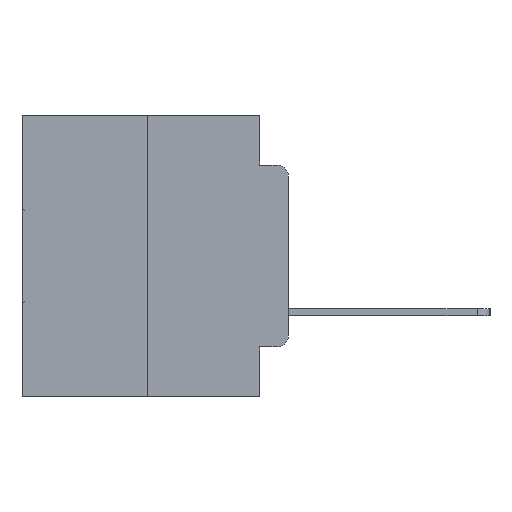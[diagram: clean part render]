
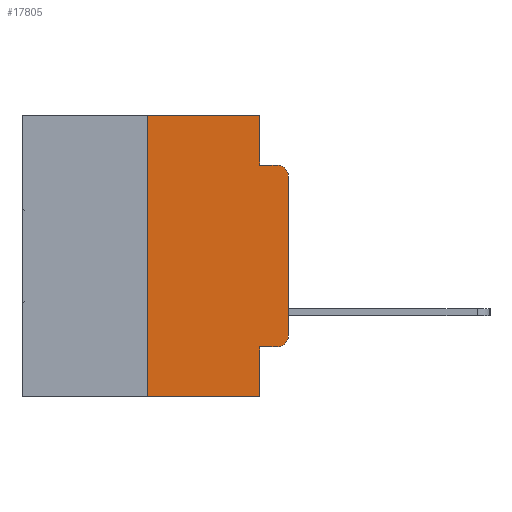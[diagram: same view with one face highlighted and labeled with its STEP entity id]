
A CAD part, left-side view. The second image highlights one B-rep face of the part: STEP entity #17805.
In plain terms, the highlighted planar face has unit normal (-1, 0, 0).
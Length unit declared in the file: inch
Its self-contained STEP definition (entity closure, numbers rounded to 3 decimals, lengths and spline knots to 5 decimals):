
#22 = DIRECTION ( 'NONE',  ( 0., -1., 0. ) ) ;
#305 = EDGE_CURVE ( 'NONE', #5735, #584, #22031, .T. ) ;
#584 = VERTEX_POINT ( 'NONE', #6001 ) ;
#732 = CARTESIAN_POINT ( 'NONE',  ( 0., 0., 0. ) ) ;
#795 = DIRECTION ( 'NONE',  ( 0., 0., -1. ) ) ;
#1579 = LINE ( 'NONE', #11698, #13246 ) ;
#1868 = DIRECTION ( 'NONE',  ( 0., 0., -1. ) ) ;
#2192 = CARTESIAN_POINT ( 'NONE',  ( 0., 0.051, -0.4115 ) ) ;
#2317 = EDGE_CURVE ( 'NONE', #20866, #5735, #18173, .T. ) ;
#2968 = VERTEX_POINT ( 'NONE', #26319 ) ;
#3524 = DIRECTION ( 'NONE',  ( 0., -1., 0. ) ) ;
#3721 = VECTOR ( 'NONE', #23520, 39.37008 ) ;
#3777 = AXIS2_PLACEMENT_3D ( 'NONE', #26623, #26662, #23555 ) ;
#3872 = EDGE_CURVE ( 'NONE', #2968, #20866, #18492, .T. ) ;
#4192 = CARTESIAN_POINT ( 'NONE',  ( 0., 0.051, 0. ) ) ;
#4450 = VERTEX_POINT ( 'NONE', #26108 ) ;
#4861 = DIRECTION ( 'NONE',  ( 0., 0., -1. ) ) ;
#5100 = LINE ( 'NONE', #16419, #10590 ) ;
#5735 = VERTEX_POINT ( 'NONE', #8322 ) ;
#6001 = CARTESIAN_POINT ( 'NONE',  ( 0., 0., -0.1085 ) ) ;
#6423 = AXIS2_PLACEMENT_3D ( 'NONE', #16955, #14727, #795 ) ;
#6938 = CARTESIAN_POINT ( 'NONE',  ( 0., 0.051, -0.5 ) ) ;
#7175 = EDGE_LOOP ( 'NONE', ( #10568, #18130, #8003, #26688, #22268, #17783, #13132, #14548, #16024, #17432 ) ) ;
#7553 = EDGE_CURVE ( 'NONE', #26560, #16601, #14676, .T. ) ;
#7652 = CARTESIAN_POINT ( 'NONE',  ( 0., 0.473, 0. ) ) ;
#7906 = AXIS2_PLACEMENT_3D ( 'NONE', #28959, #15793, #1868 ) ;
#8003 = ORIENTED_EDGE ( 'NONE', *, *, #7553, .F. ) ;
#8322 = CARTESIAN_POINT ( 'NONE',  ( 0., 0., -0.3915 ) ) ;
#9717 = CARTESIAN_POINT ( 'NONE',  ( 0., 0.25, 0. ) ) ;
#9956 = VECTOR ( 'NONE', #24204, 39.37008 ) ;
#10568 = ORIENTED_EDGE ( 'NONE', *, *, #305, .T. ) ;
#10590 = VECTOR ( 'NONE', #4861, 39.37008 ) ;
#11087 = CARTESIAN_POINT ( 'NONE',  ( 0., 0.25, 0. ) ) ;
#11698 = CARTESIAN_POINT ( 'NONE',  ( 0., 0.473, -0.5 ) ) ;
#11951 = VECTOR ( 'NONE', #22477, 39.37008 ) ;
#12445 = PLANE ( 'NONE',  #6423 ) ;
#13132 = ORIENTED_EDGE ( 'NONE', *, *, #25888, .T. ) ;
#13246 = VECTOR ( 'NONE', #22, 39.37008 ) ;
#13635 = VECTOR ( 'NONE', #26700, 39.37008 ) ;
#14115 = LINE ( 'NONE', #4192, #11951 ) ;
#14208 = VERTEX_POINT ( 'NONE', #6938 ) ;
#14324 = LINE ( 'NONE', #11087, #13635 ) ;
#14464 = FACE_OUTER_BOUND ( 'NONE', #7175, .T. ) ;
#14548 = ORIENTED_EDGE ( 'NONE', *, *, #18091, .F. ) ;
#14676 = LINE ( 'NONE', #20909, #20699 ) ;
#14727 = DIRECTION ( 'NONE',  ( 1., 0., 0. ) ) ;
#15328 = EDGE_CURVE ( 'NONE', #584, #16601, #27439, .T. ) ;
#15566 = EDGE_CURVE ( 'NONE', #28859, #19175, #21282, .T. ) ;
#15595 = CARTESIAN_POINT ( 'NONE',  ( 0., 0.02, -0.4115 ) ) ;
#15793 = DIRECTION ( 'NONE',  ( -1., 0., 0. ) ) ;
#16024 = ORIENTED_EDGE ( 'NONE', *, *, #3872, .T. ) ;
#16362 = CARTESIAN_POINT ( 'NONE',  ( 0., 0.051, -0.0885 ) ) ;
#16419 = CARTESIAN_POINT ( 'NONE',  ( 0., 0.051, 0. ) ) ;
#16601 = VERTEX_POINT ( 'NONE', #27849 ) ;
#16955 = CARTESIAN_POINT ( 'NONE',  ( 0., 0.473, 0. ) ) ;
#17432 = ORIENTED_EDGE ( 'NONE', *, *, #2317, .T. ) ;
#17783 = ORIENTED_EDGE ( 'NONE', *, *, #25730, .F. ) ;
#17792 = VECTOR ( 'NONE', #3524, 39.37008 ) ;
#17805 = ADVANCED_FACE ( 'NONE', ( #14464 ), #12445, .F. ) ;
#18091 = EDGE_CURVE ( 'NONE', #2968, #14208, #14115, .T. ) ;
#18130 = ORIENTED_EDGE ( 'NONE', *, *, #15328, .T. ) ;
#18172 = CARTESIAN_POINT ( 'NONE',  ( 0., 0.051, 0. ) ) ;
#18173 = CIRCLE ( 'NONE', #3777, 0.02 ) ;
#18492 = LINE ( 'NONE', #2192, #17792 ) ;
#19175 = VERTEX_POINT ( 'NONE', #18172 ) ;
#20699 = VECTOR ( 'NONE', #20820, 39.37008 ) ;
#20820 = DIRECTION ( 'NONE',  ( 0., -1., 0. ) ) ;
#20866 = VERTEX_POINT ( 'NONE', #15595 ) ;
#20909 = CARTESIAN_POINT ( 'NONE',  ( 0., 0.051, -0.0885 ) ) ;
#21282 = LINE ( 'NONE', #7652, #3721 ) ;
#22031 = LINE ( 'NONE', #732, #9956 ) ;
#22268 = ORIENTED_EDGE ( 'NONE', *, *, #15566, .F. ) ;
#22477 = DIRECTION ( 'NONE',  ( 0., 0., -1. ) ) ;
#23520 = DIRECTION ( 'NONE',  ( 0., -1., 0. ) ) ;
#23555 = DIRECTION ( 'NONE',  ( 0., 0., -1. ) ) ;
#24204 = DIRECTION ( 'NONE',  ( 0., 0., 1. ) ) ;
#25730 = EDGE_CURVE ( 'NONE', #4450, #28859, #14324, .T. ) ;
#25888 = EDGE_CURVE ( 'NONE', #4450, #14208, #1579, .T. ) ;
#26108 = CARTESIAN_POINT ( 'NONE',  ( 0., 0.25, -0.5 ) ) ;
#26319 = CARTESIAN_POINT ( 'NONE',  ( 0., 0.051, -0.4115 ) ) ;
#26560 = VERTEX_POINT ( 'NONE', #16362 ) ;
#26623 = CARTESIAN_POINT ( 'NONE',  ( 0., 0.02, -0.3915 ) ) ;
#26662 = DIRECTION ( 'NONE',  ( -1., 0., 0. ) ) ;
#26688 = ORIENTED_EDGE ( 'NONE', *, *, #27192, .F. ) ;
#26700 = DIRECTION ( 'NONE',  ( 0., 0., 1. ) ) ;
#27192 = EDGE_CURVE ( 'NONE', #19175, #26560, #5100, .T. ) ;
#27439 = CIRCLE ( 'NONE', #7906, 0.02 ) ;
#27849 = CARTESIAN_POINT ( 'NONE',  ( 0., 0.02, -0.0885 ) ) ;
#28859 = VERTEX_POINT ( 'NONE', #9717 ) ;
#28959 = CARTESIAN_POINT ( 'NONE',  ( 0., 0.02, -0.1085 ) ) ;
